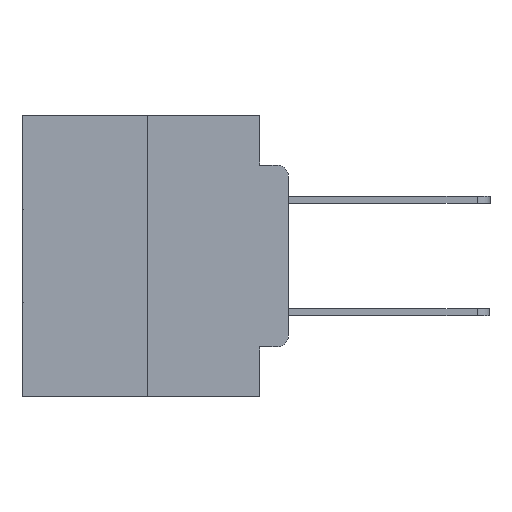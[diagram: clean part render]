
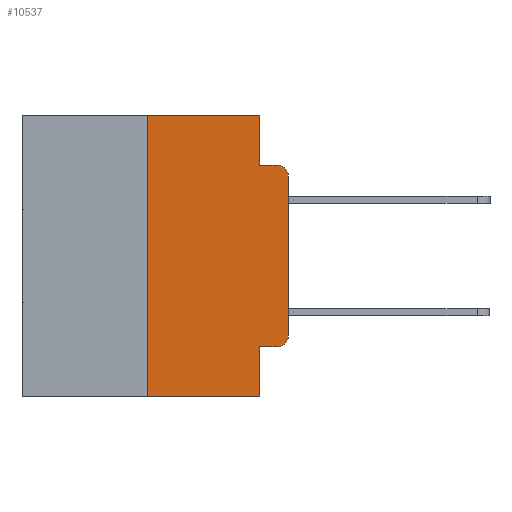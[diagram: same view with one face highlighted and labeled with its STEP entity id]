
A CAD part, left-side view. The second image highlights one B-rep face of the part: STEP entity #10537.
In plain terms, the highlighted planar face has unit normal (-1, 0, 0).
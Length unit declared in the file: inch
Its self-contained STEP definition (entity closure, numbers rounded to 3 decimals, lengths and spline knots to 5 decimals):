
#640 = VECTOR ( 'NONE', #9417, 39.37008 ) ;
#815 = CARTESIAN_POINT ( 'NONE',  ( 0., 0.473, 0. ) ) ;
#950 = ORIENTED_EDGE ( 'NONE', *, *, #5949, .T. ) ;
#1169 = VERTEX_POINT ( 'NONE', #13483 ) ;
#1435 = DIRECTION ( 'NONE',  ( 0., -1., 0. ) ) ;
#1546 = EDGE_CURVE ( 'NONE', #6571, #25069, #25715, .T. ) ;
#2000 = EDGE_LOOP ( 'NONE', ( #24751, #18450, #8074, #20483, #22484, #12276, #950, #15067, #17798, #16441 ) ) ;
#2335 = CIRCLE ( 'NONE', #6000, 0.02 ) ;
#2560 = EDGE_CURVE ( 'NONE', #1169, #13778, #2335, .T. ) ;
#2856 = LINE ( 'NONE', #14312, #14109 ) ;
#3112 = VECTOR ( 'NONE', #13331, 39.37008 ) ;
#3311 = LINE ( 'NONE', #815, #18968 ) ;
#3688 = VECTOR ( 'NONE', #9730, 39.37008 ) ;
#3694 = EDGE_CURVE ( 'NONE', #25816, #14054, #7594, .T. ) ;
#3793 = VECTOR ( 'NONE', #1435, 39.37008 ) ;
#4108 = EDGE_CURVE ( 'NONE', #14054, #1169, #21339, .T. ) ;
#4110 = CARTESIAN_POINT ( 'NONE',  ( 0., 0.051, -0.4115 ) ) ;
#4406 = CARTESIAN_POINT ( 'NONE',  ( 0., 0., -0.3915 ) ) ;
#4497 = LINE ( 'NONE', #27710, #3793 ) ;
#4695 = LINE ( 'NONE', #22285, #27872 ) ;
#5380 = DIRECTION ( 'NONE',  ( 0., 0., -1. ) ) ;
#5949 = EDGE_CURVE ( 'NONE', #6571, #13257, #2856, .T. ) ;
#6000 = AXIS2_PLACEMENT_3D ( 'NONE', #24625, #24415, #25087 ) ;
#6571 = VERTEX_POINT ( 'NONE', #14469 ) ;
#6706 = EDGE_CURVE ( 'NONE', #28462, #25816, #4497, .T. ) ;
#7167 = CARTESIAN_POINT ( 'NONE',  ( 0., 0.051, 0. ) ) ;
#7594 = CIRCLE ( 'NONE', #24888, 0.02 ) ;
#8074 = ORIENTED_EDGE ( 'NONE', *, *, #26585, .F. ) ;
#8084 = VECTOR ( 'NONE', #5380, 39.37008 ) ;
#8652 = PLANE ( 'NONE',  #23248 ) ;
#8822 = CARTESIAN_POINT ( 'NONE',  ( 0., 0.02, -0.3915 ) ) ;
#9177 = DIRECTION ( 'NONE',  ( 0., -1., 0. ) ) ;
#9417 = DIRECTION ( 'NONE',  ( 0., 0., -1. ) ) ;
#9634 = DIRECTION ( 'NONE',  ( 0., 0., -1. ) ) ;
#9730 = DIRECTION ( 'NONE',  ( 0., 0., 1. ) ) ;
#10537 = ADVANCED_FACE ( 'NONE', ( #26837 ), #8652, .F. ) ;
#10882 = DIRECTION ( 'NONE',  ( 1., 0., 0. ) ) ;
#12276 = ORIENTED_EDGE ( 'NONE', *, *, #1546, .F. ) ;
#12782 = CARTESIAN_POINT ( 'NONE',  ( 0., 0.051, -0.0885 ) ) ;
#13140 = CARTESIAN_POINT ( 'NONE',  ( 0., 0., 0. ) ) ;
#13257 = VERTEX_POINT ( 'NONE', #22481 ) ;
#13331 = DIRECTION ( 'NONE',  ( 0., 0., 1. ) ) ;
#13483 = CARTESIAN_POINT ( 'NONE',  ( 0., 0., -0.1085 ) ) ;
#13652 = EDGE_CURVE ( 'NONE', #23399, #14547, #14112, .T. ) ;
#13778 = VERTEX_POINT ( 'NONE', #18985 ) ;
#14054 = VERTEX_POINT ( 'NONE', #4406 ) ;
#14109 = VECTOR ( 'NONE', #27094, 39.37008 ) ;
#14112 = LINE ( 'NONE', #7167, #640 ) ;
#14312 = CARTESIAN_POINT ( 'NONE',  ( 0., 0.473, -0.5 ) ) ;
#14367 = DIRECTION ( 'NONE',  ( 0., -1., 0. ) ) ;
#14469 = CARTESIAN_POINT ( 'NONE',  ( 0., 0.25, -0.5 ) ) ;
#14547 = VERTEX_POINT ( 'NONE', #12782 ) ;
#15067 = ORIENTED_EDGE ( 'NONE', *, *, #15688, .F. ) ;
#15688 = EDGE_CURVE ( 'NONE', #28462, #13257, #24758, .T. ) ;
#16441 = ORIENTED_EDGE ( 'NONE', *, *, #3694, .T. ) ;
#17149 = CARTESIAN_POINT ( 'NONE',  ( 0., 0.02, -0.4115 ) ) ;
#17556 = DIRECTION ( 'NONE',  ( -1., 0., 0. ) ) ;
#17798 = ORIENTED_EDGE ( 'NONE', *, *, #6706, .T. ) ;
#18450 = ORIENTED_EDGE ( 'NONE', *, *, #2560, .T. ) ;
#18904 = CARTESIAN_POINT ( 'NONE',  ( 0., 0.25, 0. ) ) ;
#18968 = VECTOR ( 'NONE', #14367, 39.37008 ) ;
#18985 = CARTESIAN_POINT ( 'NONE',  ( 0., 0.02, -0.0885 ) ) ;
#19167 = CARTESIAN_POINT ( 'NONE',  ( 0., 0.25, 0. ) ) ;
#20483 = ORIENTED_EDGE ( 'NONE', *, *, #13652, .F. ) ;
#20766 = CARTESIAN_POINT ( 'NONE',  ( 0., 0.051, 0. ) ) ;
#21339 = LINE ( 'NONE', #13140, #3688 ) ;
#21718 = CARTESIAN_POINT ( 'NONE',  ( 0., 0.051, 0. ) ) ;
#22285 = CARTESIAN_POINT ( 'NONE',  ( 0., 0.051, -0.0885 ) ) ;
#22481 = CARTESIAN_POINT ( 'NONE',  ( 0., 0.051, -0.5 ) ) ;
#22484 = ORIENTED_EDGE ( 'NONE', *, *, #26296, .F. ) ;
#23248 = AXIS2_PLACEMENT_3D ( 'NONE', #23882, #10882, #25993 ) ;
#23399 = VERTEX_POINT ( 'NONE', #21718 ) ;
#23882 = CARTESIAN_POINT ( 'NONE',  ( 0., 0.473, 0. ) ) ;
#24415 = DIRECTION ( 'NONE',  ( -1., 0., 0. ) ) ;
#24625 = CARTESIAN_POINT ( 'NONE',  ( 0., 0.02, -0.1085 ) ) ;
#24751 = ORIENTED_EDGE ( 'NONE', *, *, #4108, .T. ) ;
#24758 = LINE ( 'NONE', #20766, #8084 ) ;
#24888 = AXIS2_PLACEMENT_3D ( 'NONE', #8822, #17556, #9634 ) ;
#25069 = VERTEX_POINT ( 'NONE', #18904 ) ;
#25087 = DIRECTION ( 'NONE',  ( 0., 0., -1. ) ) ;
#25715 = LINE ( 'NONE', #19167, #3112 ) ;
#25816 = VERTEX_POINT ( 'NONE', #17149 ) ;
#25993 = DIRECTION ( 'NONE',  ( 0., 0., -1. ) ) ;
#26296 = EDGE_CURVE ( 'NONE', #25069, #23399, #3311, .T. ) ;
#26585 = EDGE_CURVE ( 'NONE', #14547, #13778, #4695, .T. ) ;
#26837 = FACE_OUTER_BOUND ( 'NONE', #2000, .T. ) ;
#27094 = DIRECTION ( 'NONE',  ( 0., -1., 0. ) ) ;
#27710 = CARTESIAN_POINT ( 'NONE',  ( 0., 0.051, -0.4115 ) ) ;
#27872 = VECTOR ( 'NONE', #9177, 39.37008 ) ;
#28462 = VERTEX_POINT ( 'NONE', #4110 ) ;
